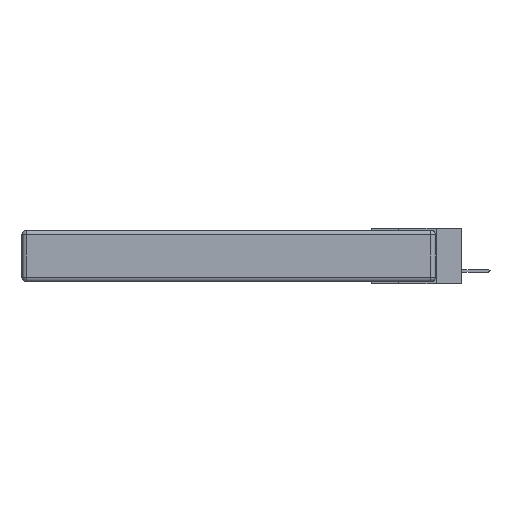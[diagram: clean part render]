
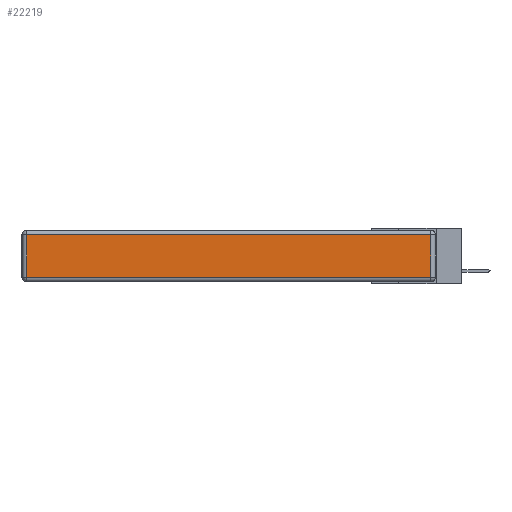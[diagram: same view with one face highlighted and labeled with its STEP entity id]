
A CAD part, left-side view. The second image highlights one B-rep face of the part: STEP entity #22219.
In plain terms, the highlighted planar face has unit normal (-1, 0, 0).
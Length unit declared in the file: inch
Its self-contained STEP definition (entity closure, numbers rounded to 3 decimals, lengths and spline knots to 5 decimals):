
#924 = VECTOR ( 'NONE', #22396, 39.37008 ) ;
#1888 = CARTESIAN_POINT ( 'NONE',  ( 0., 0.03, -0.03 ) ) ;
#4115 = ORIENTED_EDGE ( 'NONE', *, *, #14487, .T. ) ;
#6720 = CARTESIAN_POINT ( 'NONE',  ( 0., 0.03, -0.313 ) ) ;
#6735 = CARTESIAN_POINT ( 'NONE',  ( 0., 2.72, -0.03 ) ) ;
#6870 = ORIENTED_EDGE ( 'NONE', *, *, #13671, .T. ) ;
#7409 = ORIENTED_EDGE ( 'NONE', *, *, #14003, .T. ) ;
#7745 = LINE ( 'NONE', #13082, #15589 ) ;
#8503 = EDGE_LOOP ( 'NONE', ( #6870, #9595, #4115, #7409 ) ) ;
#8792 = LINE ( 'NONE', #19617, #924 ) ;
#9595 = ORIENTED_EDGE ( 'NONE', *, *, #17083, .T. ) ;
#9823 = CARTESIAN_POINT ( 'NONE',  ( 0., 0., -0.343 ) ) ;
#10564 = AXIS2_PLACEMENT_3D ( 'NONE', #9823, #28067, #12256 ) ;
#12099 = FACE_OUTER_BOUND ( 'NONE', #8503, .T. ) ;
#12147 = PLANE ( 'NONE',  #10564 ) ;
#12256 = DIRECTION ( 'NONE',  ( 0., 0., 1. ) ) ;
#12902 = LINE ( 'NONE', #32601, #15365 ) ;
#13082 = CARTESIAN_POINT ( 'NONE',  ( 0., 0.03, -0.343 ) ) ;
#13520 = CARTESIAN_POINT ( 'NONE',  ( 0., 2.75, -0.03 ) ) ;
#13671 = EDGE_CURVE ( 'NONE', #23941, #17515, #8792, .T. ) ;
#14003 = EDGE_CURVE ( 'NONE', #33316, #23941, #12902, .T. ) ;
#14487 = EDGE_CURVE ( 'NONE', #27790, #33316, #25668, .T. ) ;
#15365 = VECTOR ( 'NONE', #21967, 39.37008 ) ;
#15589 = VECTOR ( 'NONE', #26697, 39.37008 ) ;
#16391 = DIRECTION ( 'NONE',  ( 0., 1., 0. ) ) ;
#17083 = EDGE_CURVE ( 'NONE', #17515, #27790, #7745, .T. ) ;
#17515 = VERTEX_POINT ( 'NONE', #6720 ) ;
#19617 = CARTESIAN_POINT ( 'NONE',  ( 0., 0., -0.313 ) ) ;
#20671 = VECTOR ( 'NONE', #16391, 39.37008 ) ;
#21967 = DIRECTION ( 'NONE',  ( 0., 0., -1. ) ) ;
#22219 = ADVANCED_FACE ( 'NONE', ( #12099 ), #12147, .T. ) ;
#22396 = DIRECTION ( 'NONE',  ( 0., -1., 0. ) ) ;
#23672 = CARTESIAN_POINT ( 'NONE',  ( 0., 2.72, -0.313 ) ) ;
#23941 = VERTEX_POINT ( 'NONE', #23672 ) ;
#25668 = LINE ( 'NONE', #13520, #20671 ) ;
#26697 = DIRECTION ( 'NONE',  ( 0., 0., 1. ) ) ;
#27790 = VERTEX_POINT ( 'NONE', #1888 ) ;
#28067 = DIRECTION ( 'NONE',  ( -1., 0., 0. ) ) ;
#32601 = CARTESIAN_POINT ( 'NONE',  ( 0., 2.72, -0.343 ) ) ;
#33316 = VERTEX_POINT ( 'NONE', #6735 ) ;
